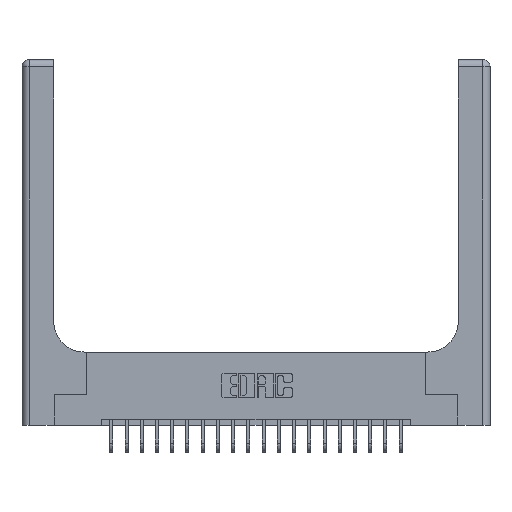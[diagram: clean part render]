
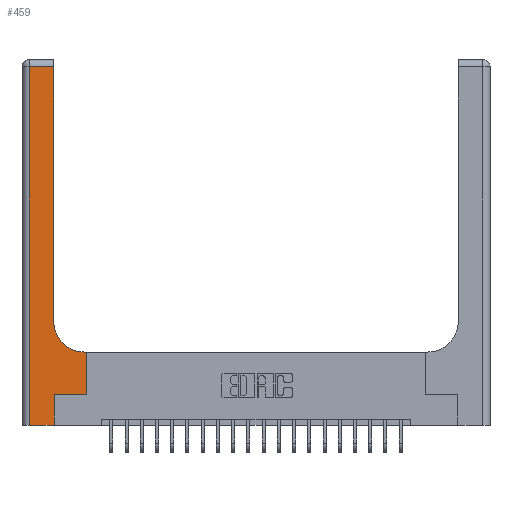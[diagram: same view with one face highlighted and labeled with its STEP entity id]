
A CAD part, top view. The second image highlights one B-rep face of the part: STEP entity #459.
In plain terms, the highlighted planar face has unit normal (0, 0, 1).
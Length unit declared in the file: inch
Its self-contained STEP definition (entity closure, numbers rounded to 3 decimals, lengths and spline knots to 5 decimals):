
#25 = EDGE_CURVE ( 'NONE', #20479, #12710, #7726, .T. ) ;
#189 = CIRCLE ( 'NONE', #2146, 0.25 ) ;
#459 = ADVANCED_FACE ( 'NONE', ( #7150 ), #2588, .F. ) ;
#1356 = ORIENTED_EDGE ( 'NONE', *, *, #5691, .T. ) ;
#1371 = VERTEX_POINT ( 'NONE', #8475 ) ;
#1720 = VERTEX_POINT ( 'NONE', #16406 ) ;
#1774 = EDGE_CURVE ( 'NONE', #18898, #20943, #6187, .T. ) ;
#2091 = CARTESIAN_POINT ( 'NONE',  ( 0.26, 0.6, 0.37 ) ) ;
#2114 = DIRECTION ( 'NONE',  ( 0., 1., 0. ) ) ;
#2117 = CARTESIAN_POINT ( 'NONE',  ( 0.26, 3., 0.37 ) ) ;
#2146 = AXIS2_PLACEMENT_3D ( 'NONE', #15776, #5092, #6857 ) ;
#2588 = PLANE ( 'NONE',  #18398 ) ;
#3087 = LINE ( 'NONE', #7215, #3910 ) ;
#3312 = CARTESIAN_POINT ( 'NONE',  ( 0.26, 2.94, 0.37 ) ) ;
#3505 = EDGE_CURVE ( 'NONE', #13221, #1720, #8328, .T. ) ;
#3910 = VECTOR ( 'NONE', #21749, 39.37008 ) ;
#4302 = VERTEX_POINT ( 'NONE', #14691 ) ;
#5092 = DIRECTION ( 'NONE',  ( 0., 0., -1. ) ) ;
#5407 = VERTEX_POINT ( 'NONE', #22195 ) ;
#5691 = EDGE_CURVE ( 'NONE', #5407, #20479, #189, .T. ) ;
#6187 = LINE ( 'NONE', #9463, #19558 ) ;
#6255 = VECTOR ( 'NONE', #22160, 39.37008 ) ;
#6857 = DIRECTION ( 'NONE',  ( 1., 0., 0. ) ) ;
#7150 = FACE_OUTER_BOUND ( 'NONE', #16800, .T. ) ;
#7215 = CARTESIAN_POINT ( 'NONE',  ( 0.528, 0.25, 0.37 ) ) ;
#7270 = CARTESIAN_POINT ( 'NONE',  ( 0.265, 0.25, 0.37 ) ) ;
#7726 = LINE ( 'NONE', #2117, #11367 ) ;
#8025 = ORIENTED_EDGE ( 'NONE', *, *, #17178, .T. ) ;
#8212 = LINE ( 'NONE', #2091, #6255 ) ;
#8328 = LINE ( 'NONE', #14271, #9707 ) ;
#8475 = CARTESIAN_POINT ( 'NONE',  ( 0.06, 2.94, 0.37 ) ) ;
#8758 = ORIENTED_EDGE ( 'NONE', *, *, #1774, .T. ) ;
#9376 = ORIENTED_EDGE ( 'NONE', *, *, #3505, .T. ) ;
#9419 = EDGE_CURVE ( 'NONE', #12710, #1371, #22249, .T. ) ;
#9463 = CARTESIAN_POINT ( 'NONE',  ( 0.265, 0.25, 0.37 ) ) ;
#9707 = VECTOR ( 'NONE', #16116, 39.37008 ) ;
#10515 = ORIENTED_EDGE ( 'NONE', *, *, #25, .T. ) ;
#11367 = VECTOR ( 'NONE', #14535, 39.37008 ) ;
#11568 = CARTESIAN_POINT ( 'NONE',  ( 0., 2.94, 0.37 ) ) ;
#11612 = CARTESIAN_POINT ( 'NONE',  ( 0.26, 0.85, 0.37 ) ) ;
#12220 = VECTOR ( 'NONE', #2114, 39.37008 ) ;
#12710 = VERTEX_POINT ( 'NONE', #3312 ) ;
#12961 = EDGE_CURVE ( 'NONE', #4302, #5407, #8212, .T. ) ;
#13112 = ORIENTED_EDGE ( 'NONE', *, *, #20883, .T. ) ;
#13221 = VERTEX_POINT ( 'NONE', #13871 ) ;
#13384 = VECTOR ( 'NONE', #18626, 39.37008 ) ;
#13779 = DIRECTION ( 'NONE',  ( 0., 0., -1. ) ) ;
#13871 = CARTESIAN_POINT ( 'NONE',  ( 0.06, 0., 0.37 ) ) ;
#14271 = CARTESIAN_POINT ( 'NONE',  ( 0., 0., 0.37 ) ) ;
#14381 = CARTESIAN_POINT ( 'NONE',  ( 0.265, 0., 0.37 ) ) ;
#14535 = DIRECTION ( 'NONE',  ( 0., 1., 0. ) ) ;
#14621 = EDGE_CURVE ( 'NONE', #1371, #13221, #16221, .T. ) ;
#14691 = CARTESIAN_POINT ( 'NONE',  ( 0.528, 0.6, 0.37 ) ) ;
#14806 = ORIENTED_EDGE ( 'NONE', *, *, #9419, .T. ) ;
#15163 = ORIENTED_EDGE ( 'NONE', *, *, #12961, .T. ) ;
#15776 = CARTESIAN_POINT ( 'NONE',  ( 0.51, 0.85, 0.37 ) ) ;
#16116 = DIRECTION ( 'NONE',  ( 1., 0., 0. ) ) ;
#16221 = LINE ( 'NONE', #21769, #17600 ) ;
#16406 = CARTESIAN_POINT ( 'NONE',  ( 0.265, 0., 0.37 ) ) ;
#16770 = ORIENTED_EDGE ( 'NONE', *, *, #14621, .T. ) ;
#16800 = EDGE_LOOP ( 'NONE', ( #10515, #14806, #16770, #9376, #8025, #8758, #13112, #15163, #1356 ) ) ;
#17178 = EDGE_CURVE ( 'NONE', #1720, #18898, #17492, .T. ) ;
#17492 = LINE ( 'NONE', #14381, #12220 ) ;
#17600 = VECTOR ( 'NONE', #18272, 39.37008 ) ;
#18272 = DIRECTION ( 'NONE',  ( 0., -1., 0. ) ) ;
#18398 = AXIS2_PLACEMENT_3D ( 'NONE', #19961, #13779, #21201 ) ;
#18626 = DIRECTION ( 'NONE',  ( -1., 0., 0. ) ) ;
#18898 = VERTEX_POINT ( 'NONE', #7270 ) ;
#19558 = VECTOR ( 'NONE', #21891, 39.37008 ) ;
#19949 = CARTESIAN_POINT ( 'NONE',  ( 0.528, 0.25, 0.37 ) ) ;
#19961 = CARTESIAN_POINT ( 'NONE',  ( 0., 3., 0.37 ) ) ;
#20479 = VERTEX_POINT ( 'NONE', #11612 ) ;
#20883 = EDGE_CURVE ( 'NONE', #20943, #4302, #3087, .T. ) ;
#20943 = VERTEX_POINT ( 'NONE', #19949 ) ;
#21201 = DIRECTION ( 'NONE',  ( -1., 0., 0. ) ) ;
#21749 = DIRECTION ( 'NONE',  ( 0., 1., 0. ) ) ;
#21769 = CARTESIAN_POINT ( 'NONE',  ( 0.06, 3., 0.37 ) ) ;
#21891 = DIRECTION ( 'NONE',  ( 1., 0., 0. ) ) ;
#22160 = DIRECTION ( 'NONE',  ( -1., 0., 0. ) ) ;
#22195 = CARTESIAN_POINT ( 'NONE',  ( 0.51, 0.6, 0.37 ) ) ;
#22249 = LINE ( 'NONE', #11568, #13384 ) ;
